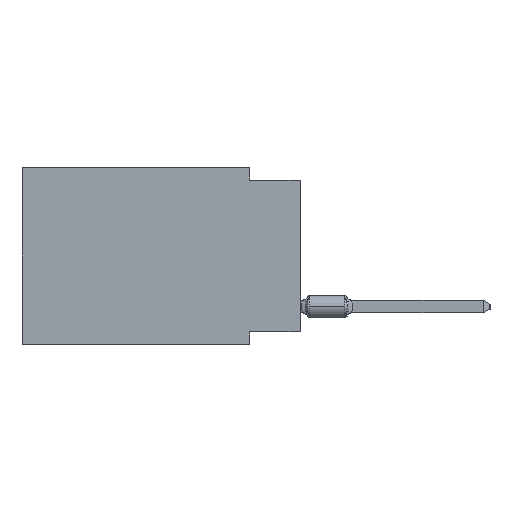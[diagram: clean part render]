
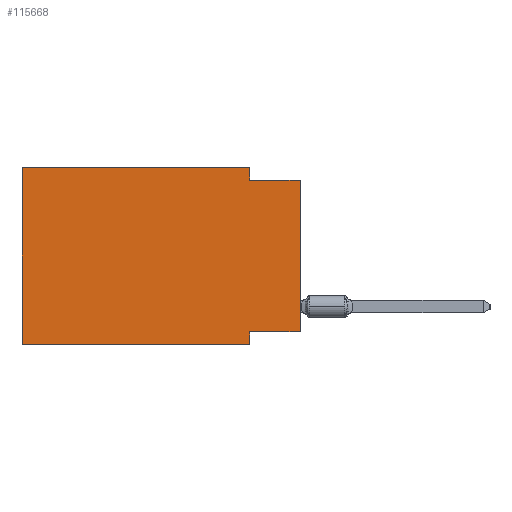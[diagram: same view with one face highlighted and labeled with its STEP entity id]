
A CAD part, left-side view. The second image highlights one B-rep face of the part: STEP entity #115668.
In plain terms, the highlighted planar face has unit normal (-1, 0, 0).
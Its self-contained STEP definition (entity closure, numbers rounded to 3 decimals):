
#1384 = VERTEX_POINT ( 'NONE', #29976 ) ;
#1485 = VERTEX_POINT ( 'NONE', #73502 ) ;
#2656 = LINE ( 'NONE', #39139, #28358 ) ;
#3688 = EDGE_CURVE ( 'NONE', #8038, #19723, #29703, .T. ) ;
#3847 = CARTESIAN_POINT ( 'NONE',  ( 0., 13.97, 0. ) ) ;
#4632 = ORIENTED_EDGE ( 'NONE', *, *, #3688, .F. ) ;
#6068 = LINE ( 'NONE', #103668, #41095 ) ;
#7707 = VECTOR ( 'NONE', #83767, 1000. ) ;
#8038 = VERTEX_POINT ( 'NONE', #17593 ) ;
#8292 = ORIENTED_EDGE ( 'NONE', *, *, #62290, .F. ) ;
#9184 = ORIENTED_EDGE ( 'NONE', *, *, #87197, .F. ) ;
#10416 = CARTESIAN_POINT ( 'NONE',  ( 0., 13.97, 0. ) ) ;
#14962 = EDGE_CURVE ( 'NONE', #80637, #1384, #34468, .T. ) ;
#17593 = CARTESIAN_POINT ( 'NONE',  ( 0., 2.54, -8.255 ) ) ;
#19001 = ORIENTED_EDGE ( 'NONE', *, *, #29369, .F. ) ;
#19723 = VERTEX_POINT ( 'NONE', #87835 ) ;
#20333 = LINE ( 'NONE', #3847, #87753 ) ;
#23360 = CARTESIAN_POINT ( 'NONE',  ( 0., 13.97, -8.89 ) ) ;
#24476 = VERTEX_POINT ( 'NONE', #23360 ) ;
#26606 = AXIS2_PLACEMENT_3D ( 'NONE', #10416, #46320, #63349 ) ;
#28358 = VECTOR ( 'NONE', #93767, 1000. ) ;
#29369 = EDGE_CURVE ( 'NONE', #86093, #1485, #20333, .T. ) ;
#29703 = LINE ( 'NONE', #65529, #94785 ) ;
#29976 = CARTESIAN_POINT ( 'NONE',  ( 0., 0., -0.635 ) ) ;
#30301 = LINE ( 'NONE', #40284, #7707 ) ;
#30872 = ORIENTED_EDGE ( 'NONE', *, *, #112411, .F. ) ;
#33291 = CARTESIAN_POINT ( 'NONE',  ( 0., 0., -0.635 ) ) ;
#33438 = DIRECTION ( 'NONE',  ( 0., 0., -1. ) ) ;
#34468 = LINE ( 'NONE', #33291, #52517 ) ;
#39139 = CARTESIAN_POINT ( 'NONE',  ( 0., 13.97, 0. ) ) ;
#40284 = CARTESIAN_POINT ( 'NONE',  ( 0., 0., 0. ) ) ;
#40905 = CARTESIAN_POINT ( 'NONE',  ( 0., 0., -8.255 ) ) ;
#41095 = VECTOR ( 'NONE', #67209, 1000. ) ;
#42865 = LINE ( 'NONE', #78683, #114371 ) ;
#45327 = VECTOR ( 'NONE', #49147, 1000. ) ;
#45746 = PLANE ( 'NONE',  #26606 ) ;
#46320 = DIRECTION ( 'NONE',  ( 1., 0., 0. ) ) ;
#49147 = DIRECTION ( 'NONE',  ( 0., 1., 0. ) ) ;
#50271 = CARTESIAN_POINT ( 'NONE',  ( 0., 13.97, 0. ) ) ;
#50961 = DIRECTION ( 'NONE',  ( 0., -1., 0. ) ) ;
#52517 = VECTOR ( 'NONE', #50961, 1000. ) ;
#55123 = FACE_OUTER_BOUND ( 'NONE', #114091, .T. ) ;
#56228 = DIRECTION ( 'NONE',  ( 0., -1., 0. ) ) ;
#62290 = EDGE_CURVE ( 'NONE', #101367, #8038, #84952, .T. ) ;
#63349 = DIRECTION ( 'NONE',  ( 0., 0., -1. ) ) ;
#65529 = CARTESIAN_POINT ( 'NONE',  ( 0., 2.54, -8.89 ) ) ;
#67209 = DIRECTION ( 'NONE',  ( 0., -1., 0. ) ) ;
#72804 = ORIENTED_EDGE ( 'NONE', *, *, #105447, .T. ) ;
#73502 = CARTESIAN_POINT ( 'NONE',  ( 0., 2.54, 0. ) ) ;
#78683 = CARTESIAN_POINT ( 'NONE',  ( 0., 2.54, 0. ) ) ;
#80637 = VERTEX_POINT ( 'NONE', #111865 ) ;
#83751 = DIRECTION ( 'NONE',  ( 0., 0., -1. ) ) ;
#83767 = DIRECTION ( 'NONE',  ( 0., 0., 1. ) ) ;
#84952 = LINE ( 'NONE', #40905, #45327 ) ;
#85484 = ORIENTED_EDGE ( 'NONE', *, *, #14962, .F. ) ;
#85898 = EDGE_CURVE ( 'NONE', #101367, #1384, #30301, .T. ) ;
#86093 = VERTEX_POINT ( 'NONE', #50271 ) ;
#86576 = CARTESIAN_POINT ( 'NONE',  ( 0., 0., -8.255 ) ) ;
#87197 = EDGE_CURVE ( 'NONE', #24476, #86093, #2656, .T. ) ;
#87753 = VECTOR ( 'NONE', #56228, 1000. ) ;
#87835 = CARTESIAN_POINT ( 'NONE',  ( 0., 2.54, -8.89 ) ) ;
#93767 = DIRECTION ( 'NONE',  ( 0., 0., 1. ) ) ;
#94785 = VECTOR ( 'NONE', #83751, 1000. ) ;
#101367 = VERTEX_POINT ( 'NONE', #86576 ) ;
#103668 = CARTESIAN_POINT ( 'NONE',  ( 0., 13.97, -8.89 ) ) ;
#105447 = EDGE_CURVE ( 'NONE', #24476, #19723, #6068, .T. ) ;
#105906 = ORIENTED_EDGE ( 'NONE', *, *, #85898, .T. ) ;
#111865 = CARTESIAN_POINT ( 'NONE',  ( 0., 2.54, -0.635 ) ) ;
#112411 = EDGE_CURVE ( 'NONE', #1485, #80637, #42865, .T. ) ;
#114091 = EDGE_LOOP ( 'NONE', ( #105906, #85484, #30872, #19001, #9184, #72804, #4632, #8292 ) ) ;
#114371 = VECTOR ( 'NONE', #33438, 1000. ) ;
#115668 = ADVANCED_FACE ( 'NONE', ( #55123 ), #45746, .F. ) ;
